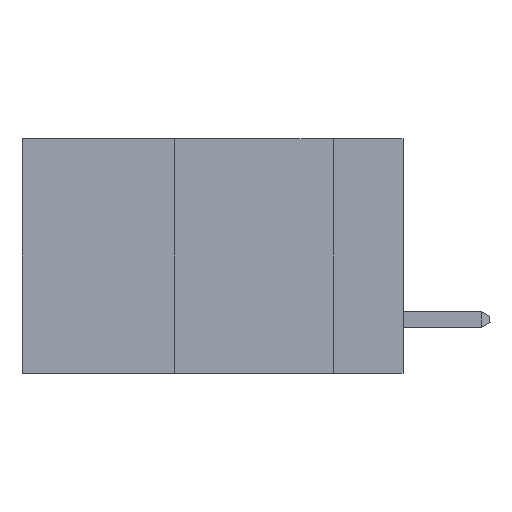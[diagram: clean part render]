
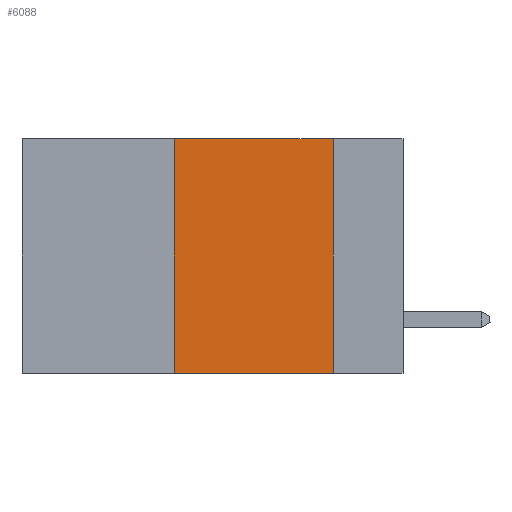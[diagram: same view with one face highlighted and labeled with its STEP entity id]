
A CAD part, left-side view. The second image highlights one B-rep face of the part: STEP entity #6088.
In plain terms, the highlighted planar face has unit normal (-1, 0, 0).
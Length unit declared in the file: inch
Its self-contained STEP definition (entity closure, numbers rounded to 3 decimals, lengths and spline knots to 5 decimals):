
#1231 = VECTOR ( 'NONE', #16981, 39.37008 ) ;
#4258 = CARTESIAN_POINT ( 'NONE',  ( 0., 0.36, -0.37 ) ) ;
#4521 = EDGE_CURVE ( 'NONE', #13248, #18673, #25557, .T. ) ;
#4709 = LINE ( 'NONE', #14188, #27067 ) ;
#5061 = ORIENTED_EDGE ( 'NONE', *, *, #22132, .F. ) ;
#5776 = VECTOR ( 'NONE', #16932, 39.37008 ) ;
#6088 = ADVANCED_FACE ( 'NONE', ( #24197 ), #8651, .F. ) ;
#7696 = EDGE_CURVE ( 'NONE', #15995, #18673, #16931, .T. ) ;
#8004 = CARTESIAN_POINT ( 'NONE',  ( 0., 0.11, 0. ) ) ;
#8305 = CARTESIAN_POINT ( 'NONE',  ( 0., 0.6, -0.37 ) ) ;
#8470 = CARTESIAN_POINT ( 'NONE',  ( 0., 0.6, 0. ) ) ;
#8651 = PLANE ( 'NONE',  #21301 ) ;
#9035 = LINE ( 'NONE', #10468, #1231 ) ;
#9381 = ORIENTED_EDGE ( 'NONE', *, *, #15269, .F. ) ;
#10468 = CARTESIAN_POINT ( 'NONE',  ( 0., 0.36, 0. ) ) ;
#13248 = VERTEX_POINT ( 'NONE', #8004 ) ;
#14188 = CARTESIAN_POINT ( 'NONE',  ( 0., 0.6, 0. ) ) ;
#14614 = CARTESIAN_POINT ( 'NONE',  ( 0., 0.11, -0.37 ) ) ;
#14719 = DIRECTION ( 'NONE',  ( 1., 0., 0. ) ) ;
#15269 = EDGE_CURVE ( 'NONE', #15995, #24934, #9035, .T. ) ;
#15995 = VERTEX_POINT ( 'NONE', #4258 ) ;
#16931 = LINE ( 'NONE', #8305, #5776 ) ;
#16932 = DIRECTION ( 'NONE',  ( 0., -1., 0. ) ) ;
#16981 = DIRECTION ( 'NONE',  ( 0., 0., 1. ) ) ;
#17054 = ORIENTED_EDGE ( 'NONE', *, *, #4521, .F. ) ;
#18673 = VERTEX_POINT ( 'NONE', #14614 ) ;
#19210 = DIRECTION ( 'NONE',  ( 0., 0., -1. ) ) ;
#20921 = DIRECTION ( 'NONE',  ( 0., 0., -1. ) ) ;
#20931 = CARTESIAN_POINT ( 'NONE',  ( 0., 0.36, 0. ) ) ;
#21206 = VECTOR ( 'NONE', #20921, 39.37008 ) ;
#21301 = AXIS2_PLACEMENT_3D ( 'NONE', #8470, #14719, #19210 ) ;
#21646 = EDGE_LOOP ( 'NONE', ( #17054, #5061, #9381, #21915 ) ) ;
#21915 = ORIENTED_EDGE ( 'NONE', *, *, #7696, .T. ) ;
#22132 = EDGE_CURVE ( 'NONE', #24934, #13248, #4709, .T. ) ;
#23054 = DIRECTION ( 'NONE',  ( 0., -1., 0. ) ) ;
#23471 = CARTESIAN_POINT ( 'NONE',  ( 0., 0.11, 0. ) ) ;
#24197 = FACE_OUTER_BOUND ( 'NONE', #21646, .T. ) ;
#24934 = VERTEX_POINT ( 'NONE', #20931 ) ;
#25557 = LINE ( 'NONE', #23471, #21206 ) ;
#27067 = VECTOR ( 'NONE', #23054, 39.37008 ) ;
